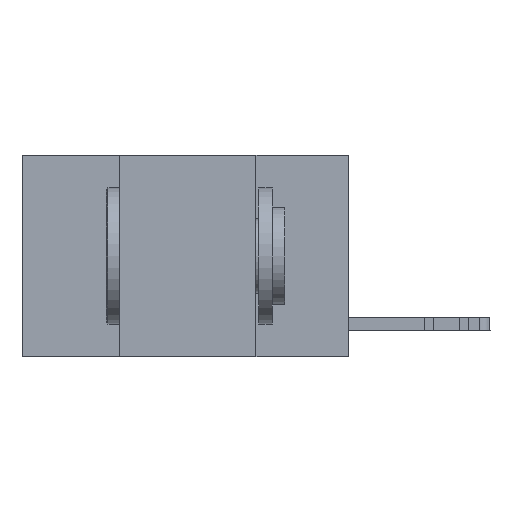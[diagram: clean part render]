
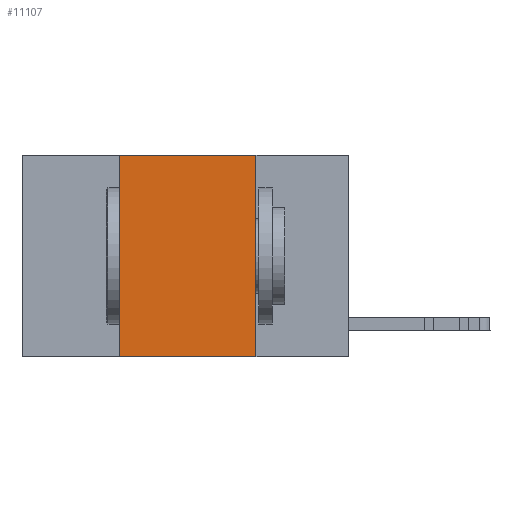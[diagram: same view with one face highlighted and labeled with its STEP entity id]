
A CAD part, left-side view. The second image highlights one B-rep face of the part: STEP entity #11107.
In plain terms, the highlighted planar face has unit normal (-1, 0, 0).
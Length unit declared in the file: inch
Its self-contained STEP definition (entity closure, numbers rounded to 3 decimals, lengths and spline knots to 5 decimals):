
#888 = VERTEX_POINT ( 'NONE', #3097 ) ;
#1595 = EDGE_CURVE ( 'NONE', #7873, #3144, #20069, .T. ) ;
#1620 = ORIENTED_EDGE ( 'NONE', *, *, #1595, .F. ) ;
#2578 = VECTOR ( 'NONE', #6097, 39.37008 ) ;
#2646 = LINE ( 'NONE', #9274, #9117 ) ;
#3097 = CARTESIAN_POINT ( 'NONE',  ( 0., 0.42, -0.37 ) ) ;
#3144 = VERTEX_POINT ( 'NONE', #9048 ) ;
#4128 = CARTESIAN_POINT ( 'NONE',  ( 0., 0.6, 0. ) ) ;
#4821 = CARTESIAN_POINT ( 'NONE',  ( 0., 0.6, -0.37 ) ) ;
#6097 = DIRECTION ( 'NONE',  ( 0., -1., 0. ) ) ;
#6597 = VECTOR ( 'NONE', #13690, 39.37008 ) ;
#7066 = AXIS2_PLACEMENT_3D ( 'NONE', #19808, #22331, #13477 ) ;
#7517 = ORIENTED_EDGE ( 'NONE', *, *, #10331, .F. ) ;
#7873 = VERTEX_POINT ( 'NONE', #19818 ) ;
#9048 = CARTESIAN_POINT ( 'NONE',  ( 0., 0.17, 0. ) ) ;
#9117 = VECTOR ( 'NONE', #16635, 39.37008 ) ;
#9274 = CARTESIAN_POINT ( 'NONE',  ( 0., 0.17, 0. ) ) ;
#10331 = EDGE_CURVE ( 'NONE', #888, #7873, #15702, .T. ) ;
#10638 = PLANE ( 'NONE',  #7066 ) ;
#11107 = ADVANCED_FACE ( 'NONE', ( #22047 ), #10638, .F. ) ;
#12191 = VECTOR ( 'NONE', #18252, 39.37008 ) ;
#13071 = EDGE_LOOP ( 'NONE', ( #21930, #1620, #7517, #21146 ) ) ;
#13477 = DIRECTION ( 'NONE',  ( 0., 0., -1. ) ) ;
#13690 = DIRECTION ( 'NONE',  ( 0., -1., 0. ) ) ;
#15702 = LINE ( 'NONE', #15848, #12191 ) ;
#15848 = CARTESIAN_POINT ( 'NONE',  ( 0., 0.42, 0. ) ) ;
#16635 = DIRECTION ( 'NONE',  ( 0., 0., -1. ) ) ;
#16805 = VERTEX_POINT ( 'NONE', #27048 ) ;
#18252 = DIRECTION ( 'NONE',  ( 0., 0., 1. ) ) ;
#19808 = CARTESIAN_POINT ( 'NONE',  ( 0., 0.6, 0. ) ) ;
#19818 = CARTESIAN_POINT ( 'NONE',  ( 0., 0.42, 0. ) ) ;
#20069 = LINE ( 'NONE', #4128, #2578 ) ;
#20383 = EDGE_CURVE ( 'NONE', #888, #16805, #25103, .T. ) ;
#21146 = ORIENTED_EDGE ( 'NONE', *, *, #20383, .T. ) ;
#21930 = ORIENTED_EDGE ( 'NONE', *, *, #22736, .F. ) ;
#22047 = FACE_OUTER_BOUND ( 'NONE', #13071, .T. ) ;
#22331 = DIRECTION ( 'NONE',  ( 1., 0., 0. ) ) ;
#22736 = EDGE_CURVE ( 'NONE', #3144, #16805, #2646, .T. ) ;
#25103 = LINE ( 'NONE', #4821, #6597 ) ;
#27048 = CARTESIAN_POINT ( 'NONE',  ( 0., 0.17, -0.37 ) ) ;
